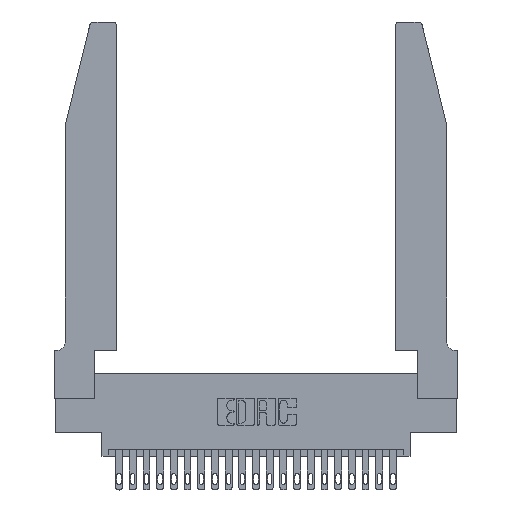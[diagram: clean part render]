
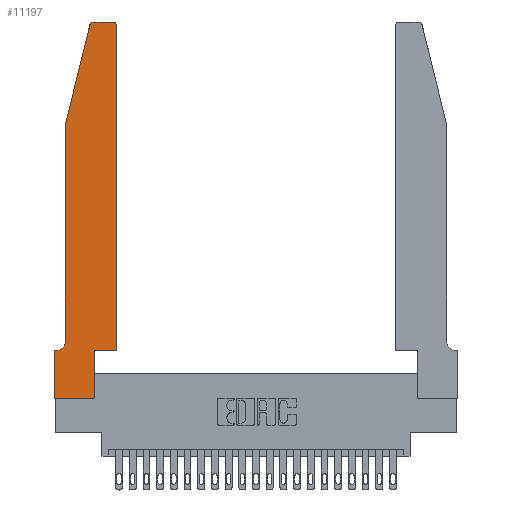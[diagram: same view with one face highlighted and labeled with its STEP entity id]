
A CAD part, top view. The second image highlights one B-rep face of the part: STEP entity #11197.
In plain terms, the highlighted planar face has unit normal (0, 0, 1).
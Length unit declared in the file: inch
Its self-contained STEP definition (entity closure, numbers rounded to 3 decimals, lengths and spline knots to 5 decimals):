
#102 = VERTEX_POINT ( 'NONE', #1014 ) ;
#108 = LINE ( 'NONE', #196, #4500 ) ;
#196 = CARTESIAN_POINT ( 'NONE',  ( 0., 0., 0.37 ) ) ;
#645 = CARTESIAN_POINT ( 'NONE',  ( 0.0755, 2., 0.37 ) ) ;
#779 = CARTESIAN_POINT ( 'NONE',  ( 0.0755, 0.35, 0.37 ) ) ;
#883 = ORIENTED_EDGE ( 'NONE', *, *, #15326, .T. ) ;
#1014 = CARTESIAN_POINT ( 'NONE',  ( 0.4505, 0.35, 0.37 ) ) ;
#1518 = LINE ( 'NONE', #8633, #5910 ) ;
#2011 = ORIENTED_EDGE ( 'NONE', *, *, #4414, .T. ) ;
#2047 = VERTEX_POINT ( 'NONE', #9590 ) ;
#2187 = DIRECTION ( 'NONE',  ( 0., 1., 0. ) ) ;
#2310 = DIRECTION ( 'NONE',  ( 1., 0., 0. ) ) ;
#2548 = EDGE_CURVE ( 'NONE', #22759, #2644, #18031, .T. ) ;
#2644 = VERTEX_POINT ( 'NONE', #15200 ) ;
#3143 = EDGE_CURVE ( 'NONE', #14894, #21636, #8976, .T. ) ;
#3153 = VECTOR ( 'NONE', #22816, 39.37008 ) ;
#3585 = DIRECTION ( 'NONE',  ( 1., 0., 0. ) ) ;
#3881 = DIRECTION ( 'NONE',  ( 1., 0., 0. ) ) ;
#3992 = DIRECTION ( 'NONE',  ( -1., 0., 0. ) ) ;
#4081 = ORIENTED_EDGE ( 'NONE', *, *, #3143, .T. ) ;
#4106 = VECTOR ( 'NONE', #17137, 39.37008 ) ;
#4232 = DIRECTION ( 'NONE',  ( 1., 0., 0. ) ) ;
#4300 = VECTOR ( 'NONE', #12424, 39.37008 ) ;
#4414 = EDGE_CURVE ( 'NONE', #102, #20330, #9761, .T. ) ;
#4500 = VECTOR ( 'NONE', #3881, 39.37008 ) ;
#4698 = CIRCLE ( 'NONE', #21177, 0.03 ) ;
#4719 = CARTESIAN_POINT ( 'NONE',  ( 0.0755, 2., 0.37 ) ) ;
#5187 = CARTESIAN_POINT ( 'NONE',  ( 0.284, 2.75, 0.37 ) ) ;
#5476 = ORIENTED_EDGE ( 'NONE', *, *, #13735, .T. ) ;
#5813 = CIRCLE ( 'NONE', #7206, 0.03 ) ;
#5910 = VECTOR ( 'NONE', #23127, 39.37008 ) ;
#6024 = ORIENTED_EDGE ( 'NONE', *, *, #11607, .T. ) ;
#6228 = ORIENTED_EDGE ( 'NONE', *, *, #9373, .T. ) ;
#6394 = VERTEX_POINT ( 'NONE', #12414 ) ;
#6954 = PLANE ( 'NONE',  #15705 ) ;
#7206 = AXIS2_PLACEMENT_3D ( 'NONE', #12866, #14632, #3585 ) ;
#7794 = CARTESIAN_POINT ( 'NONE',  ( 0.4505, 0.35, 0.37 ) ) ;
#7969 = DIRECTION ( 'NONE',  ( 1., 0., 0. ) ) ;
#8630 = ORIENTED_EDGE ( 'NONE', *, *, #2548, .T. ) ;
#8633 = CARTESIAN_POINT ( 'NONE',  ( 0.2865, 0.35, 0.37 ) ) ;
#8976 = LINE ( 'NONE', #15993, #4300 ) ;
#9373 = EDGE_CURVE ( 'NONE', #6394, #23592, #108, .T. ) ;
#9546 = EDGE_CURVE ( 'NONE', #11455, #102, #17581, .T. ) ;
#9590 = CARTESIAN_POINT ( 'NONE',  ( 0.25487, 2.72718, 0.37 ) ) ;
#9637 = CARTESIAN_POINT ( 'NONE',  ( 0.4205, 2.75, 0.37 ) ) ;
#9761 = LINE ( 'NONE', #15536, #17064 ) ;
#10223 = LINE ( 'NONE', #779, #4106 ) ;
#10628 = CARTESIAN_POINT ( 'NONE',  ( 0.0755, 2., 0.37 ) ) ;
#10629 = EDGE_CURVE ( 'NONE', #21636, #2047, #4698, .T. ) ;
#11197 = ADVANCED_FACE ( 'NONE', ( #13133 ), #6954, .T. ) ;
#11455 = VERTEX_POINT ( 'NONE', #23571 ) ;
#11607 = EDGE_CURVE ( 'NONE', #20569, #16067, #10223, .T. ) ;
#11899 = ORIENTED_EDGE ( 'NONE', *, *, #9546, .T. ) ;
#12058 = DIRECTION ( 'NONE',  ( 0., 0., 1. ) ) ;
#12167 = AXIS2_PLACEMENT_3D ( 'NONE', #16784, #20734, #3992 ) ;
#12212 = VECTOR ( 'NONE', #14900, 39.37008 ) ;
#12231 = CARTESIAN_POINT ( 'NONE',  ( 0., 0., 0.37 ) ) ;
#12414 = CARTESIAN_POINT ( 'NONE',  ( 0., 0., 0.37 ) ) ;
#12424 = DIRECTION ( 'NONE',  ( -1., 0., 0. ) ) ;
#12866 = CARTESIAN_POINT ( 'NONE',  ( 0.4205, 2.72, 0.37 ) ) ;
#12978 = CARTESIAN_POINT ( 'NONE',  ( 0., 0.35, 0.37 ) ) ;
#13058 = VECTOR ( 'NONE', #23485, 39.37008 ) ;
#13117 = CARTESIAN_POINT ( 'NONE',  ( 0.0055, 0.35, 0.37 ) ) ;
#13133 = FACE_OUTER_BOUND ( 'NONE', #22894, .T. ) ;
#13735 = EDGE_CURVE ( 'NONE', #2644, #20569, #23691, .T. ) ;
#13775 = EDGE_CURVE ( 'NONE', #23592, #11455, #1518, .T. ) ;
#14632 = DIRECTION ( 'NONE',  ( 0., 0., 1. ) ) ;
#14826 = CARTESIAN_POINT ( 'NONE',  ( 0.4505, 2.72, 0.37 ) ) ;
#14894 = VERTEX_POINT ( 'NONE', #9637 ) ;
#14900 = DIRECTION ( 'NONE',  ( 0., -1., 0. ) ) ;
#14983 = DIRECTION ( 'NONE',  ( 0., 0., 1. ) ) ;
#15200 = CARTESIAN_POINT ( 'NONE',  ( 0.0755, 0.42, 0.37 ) ) ;
#15326 = EDGE_CURVE ( 'NONE', #20330, #14894, #5813, .T. ) ;
#15536 = CARTESIAN_POINT ( 'NONE',  ( 0.4505, 0.35, 0.37 ) ) ;
#15705 = AXIS2_PLACEMENT_3D ( 'NONE', #23867, #14983, #7969 ) ;
#15993 = CARTESIAN_POINT ( 'NONE',  ( 0.2605, 2.75, 0.37 ) ) ;
#16067 = VERTEX_POINT ( 'NONE', #12978 ) ;
#16575 = EDGE_CURVE ( 'NONE', #16067, #6394, #23264, .T. ) ;
#16784 = CARTESIAN_POINT ( 'NONE',  ( 0.0055, 0.42, 0.37 ) ) ;
#17064 = VECTOR ( 'NONE', #2187, 39.37008 ) ;
#17137 = DIRECTION ( 'NONE',  ( -1., 0., 0. ) ) ;
#17171 = ORIENTED_EDGE ( 'NONE', *, *, #19433, .T. ) ;
#17581 = LINE ( 'NONE', #7794, #22541 ) ;
#18028 = LINE ( 'NONE', #645, #3153 ) ;
#18031 = LINE ( 'NONE', #4719, #12212 ) ;
#19322 = ORIENTED_EDGE ( 'NONE', *, *, #10629, .T. ) ;
#19433 = EDGE_CURVE ( 'NONE', #2047, #22759, #18028, .T. ) ;
#19457 = CARTESIAN_POINT ( 'NONE',  ( 0.284, 2.72, 0.37 ) ) ;
#20207 = CARTESIAN_POINT ( 'NONE',  ( 0.2865, 0., 0.37 ) ) ;
#20330 = VERTEX_POINT ( 'NONE', #14826 ) ;
#20569 = VERTEX_POINT ( 'NONE', #13117 ) ;
#20734 = DIRECTION ( 'NONE',  ( 0., 0., -1. ) ) ;
#20763 = ORIENTED_EDGE ( 'NONE', *, *, #13775, .T. ) ;
#21177 = AXIS2_PLACEMENT_3D ( 'NONE', #19457, #12058, #4232 ) ;
#21636 = VERTEX_POINT ( 'NONE', #5187 ) ;
#22541 = VECTOR ( 'NONE', #2310, 39.37008 ) ;
#22759 = VERTEX_POINT ( 'NONE', #10628 ) ;
#22816 = DIRECTION ( 'NONE',  ( -0.239, -0.971, 0. ) ) ;
#22894 = EDGE_LOOP ( 'NONE', ( #4081, #19322, #17171, #8630, #5476, #6024, #23697, #6228, #20763, #11899, #2011, #883 ) ) ;
#23127 = DIRECTION ( 'NONE',  ( 0., 1., 0. ) ) ;
#23264 = LINE ( 'NONE', #12231, #13058 ) ;
#23485 = DIRECTION ( 'NONE',  ( 0., -1., 0. ) ) ;
#23571 = CARTESIAN_POINT ( 'NONE',  ( 0.2865, 0.35, 0.37 ) ) ;
#23592 = VERTEX_POINT ( 'NONE', #20207 ) ;
#23691 = CIRCLE ( 'NONE', #12167, 0.07 ) ;
#23697 = ORIENTED_EDGE ( 'NONE', *, *, #16575, .T. ) ;
#23867 = CARTESIAN_POINT ( 'NONE',  ( 0., 0.35, 0.37 ) ) ;
